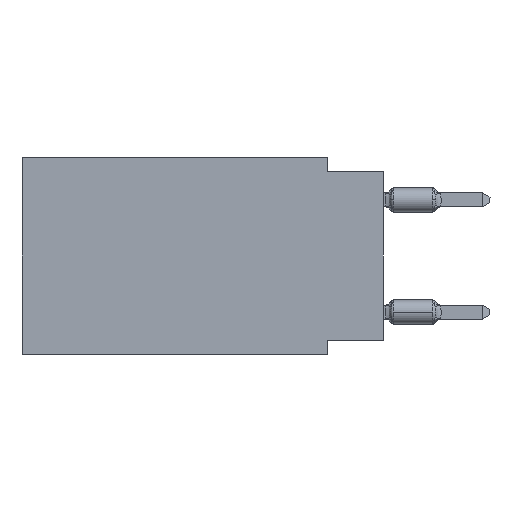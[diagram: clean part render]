
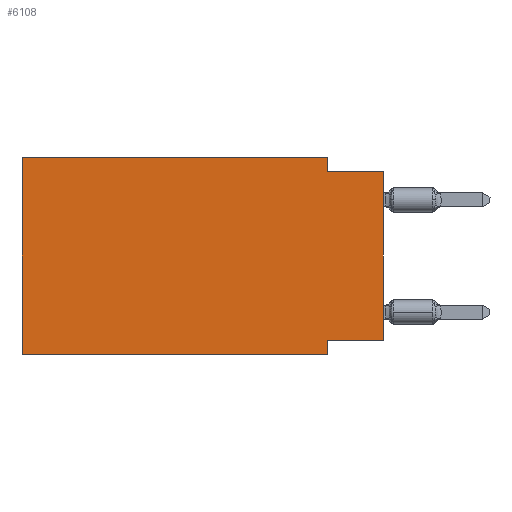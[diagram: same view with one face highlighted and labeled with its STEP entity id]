
A CAD part, left-side view. The second image highlights one B-rep face of the part: STEP entity #6108.
In plain terms, the highlighted planar face has unit normal (-1, 0, 0).
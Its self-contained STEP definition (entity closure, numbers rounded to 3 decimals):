
#505 = EDGE_CURVE ( 'NONE', #8224, #19787, #18203, .T. ) ;
#817 = EDGE_CURVE ( 'NONE', #13539, #1275, #14028, .T. ) ;
#1275 = VERTEX_POINT ( 'NONE', #4993 ) ;
#1788 = CARTESIAN_POINT ( 'NONE',  ( 0., 0., -0.635 ) ) ;
#2598 = DIRECTION ( 'NONE',  ( 1., 0., 0. ) ) ;
#2608 = EDGE_CURVE ( 'NONE', #5304, #16079, #15071, .T. ) ;
#2679 = CARTESIAN_POINT ( 'NONE',  ( 0., 2.54, -8.89 ) ) ;
#2777 = EDGE_CURVE ( 'NONE', #19292, #19787, #12014, .T. ) ;
#2848 = DIRECTION ( 'NONE',  ( 0., -1., 0. ) ) ;
#3030 = VECTOR ( 'NONE', #11641, 1000. ) ;
#3639 = VECTOR ( 'NONE', #19140, 1000. ) ;
#3661 = CARTESIAN_POINT ( 'NONE',  ( 0., 0., -0.635 ) ) ;
#4011 = CARTESIAN_POINT ( 'NONE',  ( 0., 0., -8.255 ) ) ;
#4447 = FACE_OUTER_BOUND ( 'NONE', #12191, .T. ) ;
#4993 = CARTESIAN_POINT ( 'NONE',  ( 0., 2.54, 0. ) ) ;
#5134 = ORIENTED_EDGE ( 'NONE', *, *, #2777, .F. ) ;
#5300 = DIRECTION ( 'NONE',  ( 0., 0., -1. ) ) ;
#5304 = VERTEX_POINT ( 'NONE', #16498 ) ;
#5307 = VECTOR ( 'NONE', #18045, 1000. ) ;
#5449 = CARTESIAN_POINT ( 'NONE',  ( 0., 16.383, -8.89 ) ) ;
#6108 = ADVANCED_FACE ( 'NONE', ( #4447 ), #19430, .F. ) ;
#6440 = CARTESIAN_POINT ( 'NONE',  ( 0., 16.383, -8.89 ) ) ;
#7516 = DIRECTION ( 'NONE',  ( 0., 0., -1. ) ) ;
#7630 = ORIENTED_EDGE ( 'NONE', *, *, #22777, .F. ) ;
#7636 = LINE ( 'NONE', #11089, #17138 ) ;
#7703 = LINE ( 'NONE', #4011, #3030 ) ;
#7763 = VECTOR ( 'NONE', #16321, 1000. ) ;
#8224 = VERTEX_POINT ( 'NONE', #6440 ) ;
#8518 = CARTESIAN_POINT ( 'NONE',  ( 0., 2.54, -8.89 ) ) ;
#8887 = DIRECTION ( 'NONE',  ( 0., -1., 0. ) ) ;
#9140 = VECTOR ( 'NONE', #5300, 1000. ) ;
#10105 = CARTESIAN_POINT ( 'NONE',  ( 0., 16.383, 0. ) ) ;
#10223 = LINE ( 'NONE', #17688, #5307 ) ;
#10868 = VECTOR ( 'NONE', #2848, 1000. ) ;
#11089 = CARTESIAN_POINT ( 'NONE',  ( 0., 2.54, 0. ) ) ;
#11641 = DIRECTION ( 'NONE',  ( 0., 1., 0. ) ) ;
#11657 = CARTESIAN_POINT ( 'NONE',  ( 0., 0., 0. ) ) ;
#11773 = CARTESIAN_POINT ( 'NONE',  ( 0., 2.54, -8.255 ) ) ;
#12014 = LINE ( 'NONE', #2679, #9140 ) ;
#12191 = EDGE_LOOP ( 'NONE', ( #20780, #16912, #20122, #16695, #15498, #20412, #5134, #7630 ) ) ;
#12193 = CARTESIAN_POINT ( 'NONE',  ( 0., 16.383, 0. ) ) ;
#13416 = EDGE_CURVE ( 'NONE', #8224, #13539, #10223, .T. ) ;
#13539 = VERTEX_POINT ( 'NONE', #19098 ) ;
#14028 = LINE ( 'NONE', #12193, #10868 ) ;
#14062 = AXIS2_PLACEMENT_3D ( 'NONE', #10105, #2598, #17578 ) ;
#15071 = LINE ( 'NONE', #11657, #3639 ) ;
#15330 = LINE ( 'NONE', #3661, #7763 ) ;
#15498 = ORIENTED_EDGE ( 'NONE', *, *, #13416, .F. ) ;
#15733 = EDGE_CURVE ( 'NONE', #22194, #16079, #15330, .T. ) ;
#16079 = VERTEX_POINT ( 'NONE', #1788 ) ;
#16321 = DIRECTION ( 'NONE',  ( 0., -1., 0. ) ) ;
#16472 = CARTESIAN_POINT ( 'NONE',  ( 0., 2.54, -0.635 ) ) ;
#16498 = CARTESIAN_POINT ( 'NONE',  ( 0., 0., -8.255 ) ) ;
#16695 = ORIENTED_EDGE ( 'NONE', *, *, #817, .F. ) ;
#16848 = EDGE_CURVE ( 'NONE', #1275, #22194, #7636, .T. ) ;
#16912 = ORIENTED_EDGE ( 'NONE', *, *, #15733, .F. ) ;
#17138 = VECTOR ( 'NONE', #7516, 1000. ) ;
#17578 = DIRECTION ( 'NONE',  ( 0., 0., -1. ) ) ;
#17688 = CARTESIAN_POINT ( 'NONE',  ( 0., 16.383, 0. ) ) ;
#18045 = DIRECTION ( 'NONE',  ( 0., 0., 1. ) ) ;
#18203 = LINE ( 'NONE', #5449, #20664 ) ;
#19098 = CARTESIAN_POINT ( 'NONE',  ( 0., 16.383, 0. ) ) ;
#19140 = DIRECTION ( 'NONE',  ( 0., 0., 1. ) ) ;
#19292 = VERTEX_POINT ( 'NONE', #11773 ) ;
#19430 = PLANE ( 'NONE',  #14062 ) ;
#19787 = VERTEX_POINT ( 'NONE', #8518 ) ;
#20122 = ORIENTED_EDGE ( 'NONE', *, *, #16848, .F. ) ;
#20412 = ORIENTED_EDGE ( 'NONE', *, *, #505, .T. ) ;
#20664 = VECTOR ( 'NONE', #8887, 1000. ) ;
#20780 = ORIENTED_EDGE ( 'NONE', *, *, #2608, .T. ) ;
#22194 = VERTEX_POINT ( 'NONE', #16472 ) ;
#22777 = EDGE_CURVE ( 'NONE', #5304, #19292, #7703, .T. ) ;
